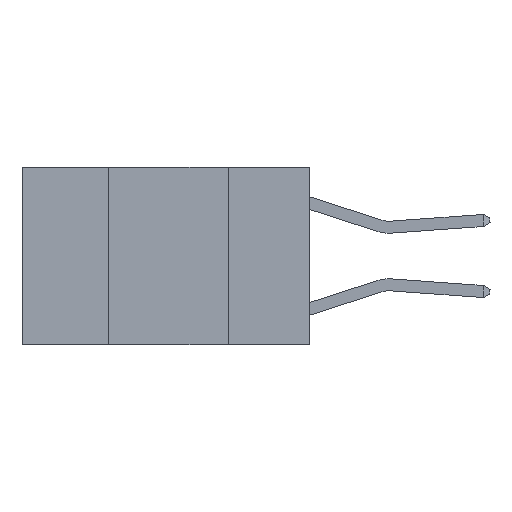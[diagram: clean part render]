
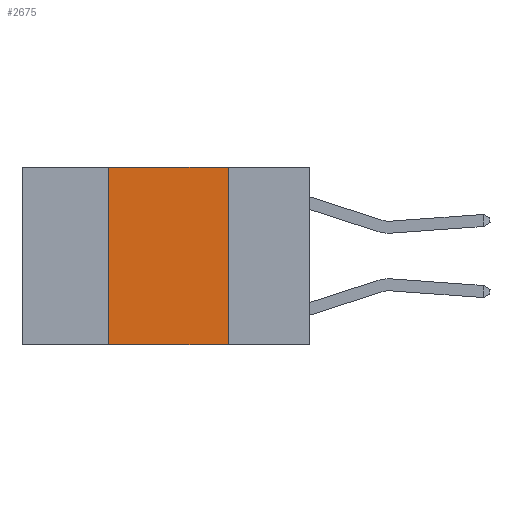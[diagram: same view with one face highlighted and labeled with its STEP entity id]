
A CAD part, left-side view. The second image highlights one B-rep face of the part: STEP entity #2675.
In plain terms, the highlighted planar face has unit normal (-1, 0, 0).
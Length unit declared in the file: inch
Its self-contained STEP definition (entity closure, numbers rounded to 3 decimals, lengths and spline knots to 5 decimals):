
#163 = VECTOR ( 'NONE', #10320, 39.37008 ) ;
#299 = DIRECTION ( 'NONE',  ( 0., -1., 0. ) ) ;
#614 = EDGE_CURVE ( 'NONE', #2536, #4286, #8111, .T. ) ;
#1492 = ORIENTED_EDGE ( 'NONE', *, *, #9839, .F. ) ;
#1537 = ORIENTED_EDGE ( 'NONE', *, *, #9845, .F. ) ;
#2326 = CARTESIAN_POINT ( 'NONE',  ( 0., 0.42, 0. ) ) ;
#2536 = VERTEX_POINT ( 'NONE', #6634 ) ;
#2675 = ADVANCED_FACE ( 'NONE', ( #3168 ), #10910, .F. ) ;
#2799 = VECTOR ( 'NONE', #299, 39.37008 ) ;
#3168 = FACE_OUTER_BOUND ( 'NONE', #9915, .T. ) ;
#4270 = DIRECTION ( 'NONE',  ( 1., 0., 0. ) ) ;
#4286 = VERTEX_POINT ( 'NONE', #6366 ) ;
#4648 = CARTESIAN_POINT ( 'NONE',  ( 0., 0.17, 0. ) ) ;
#4859 = VERTEX_POINT ( 'NONE', #4866 ) ;
#4866 = CARTESIAN_POINT ( 'NONE',  ( 0., 0.17, -0.37 ) ) ;
#5179 = LINE ( 'NONE', #9016, #2799 ) ;
#5243 = CARTESIAN_POINT ( 'NONE',  ( 0., 0.6, 0. ) ) ;
#5248 = VECTOR ( 'NONE', #8007, 39.37008 ) ;
#6232 = ORIENTED_EDGE ( 'NONE', *, *, #7690, .T. ) ;
#6366 = CARTESIAN_POINT ( 'NONE',  ( 0., 0.42, 0. ) ) ;
#6610 = DIRECTION ( 'NONE',  ( 0., 0., -1. ) ) ;
#6634 = CARTESIAN_POINT ( 'NONE',  ( 0., 0.42, -0.37 ) ) ;
#7243 = DIRECTION ( 'NONE',  ( 0., 0., -1. ) ) ;
#7373 = AXIS2_PLACEMENT_3D ( 'NONE', #5243, #4270, #7243 ) ;
#7665 = LINE ( 'NONE', #4648, #11337 ) ;
#7690 = EDGE_CURVE ( 'NONE', #2536, #4859, #5179, .T. ) ;
#8007 = DIRECTION ( 'NONE',  ( 0., 0., 1. ) ) ;
#8111 = LINE ( 'NONE', #2326, #5248 ) ;
#8541 = LINE ( 'NONE', #11362, #163 ) ;
#9016 = CARTESIAN_POINT ( 'NONE',  ( 0., 0.6, -0.37 ) ) ;
#9377 = CARTESIAN_POINT ( 'NONE',  ( 0., 0.17, 0. ) ) ;
#9839 = EDGE_CURVE ( 'NONE', #4286, #12433, #8541, .T. ) ;
#9845 = EDGE_CURVE ( 'NONE', #12433, #4859, #7665, .T. ) ;
#9915 = EDGE_LOOP ( 'NONE', ( #1537, #1492, #12472, #6232 ) ) ;
#10320 = DIRECTION ( 'NONE',  ( 0., -1., 0. ) ) ;
#10910 = PLANE ( 'NONE',  #7373 ) ;
#11337 = VECTOR ( 'NONE', #6610, 39.37008 ) ;
#11362 = CARTESIAN_POINT ( 'NONE',  ( 0., 0.6, 0. ) ) ;
#12433 = VERTEX_POINT ( 'NONE', #9377 ) ;
#12472 = ORIENTED_EDGE ( 'NONE', *, *, #614, .F. ) ;
